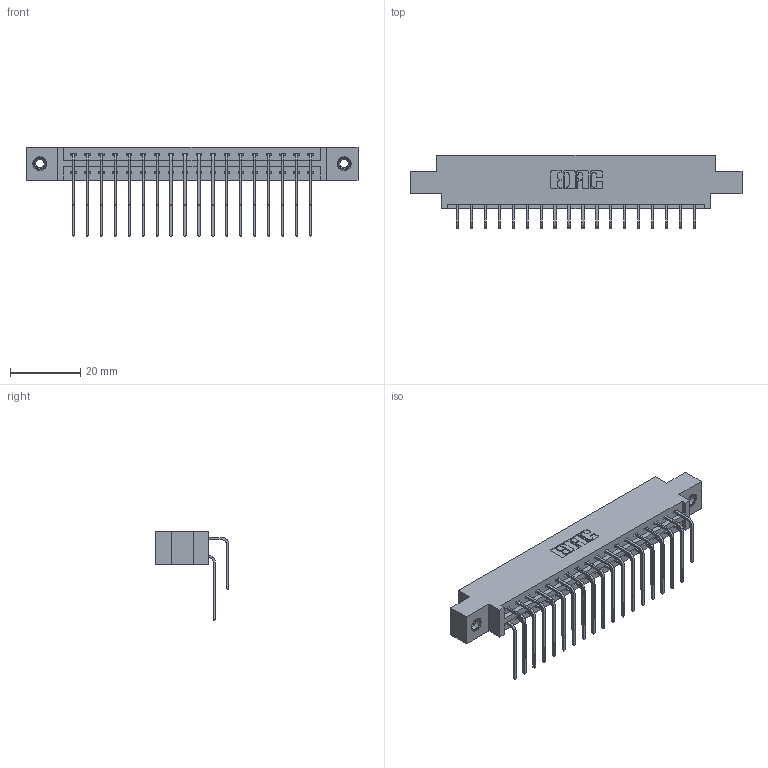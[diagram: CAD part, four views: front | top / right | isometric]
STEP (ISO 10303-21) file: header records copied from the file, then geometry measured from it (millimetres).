
FILE_DESCRIPTION (( 'STEP AP203' ), '1' );
FILE_NAME ('337-036-559-807.STEP', '2018-08-08T00:28:37', ( '' ), ( '' ), 'SwSTEP 2.0', 'SolidWorks 2016', '' );
FILE_SCHEMA (( 'CONFIG_CONTROL_DESIGN' ));
Length unit declared in the file: inch
Products named in the file (5): 337 Part_0.170 Offset - 0.156 Dia-TI; 345-292-001_558 559 Tail - 1; 345-292-001_559 Tail - 2; 345-250-001_345-250-005-103; 337-036-559-807
Assembly tree (39 placements, depth 2):
  337-036-559-807
    337 Part_0.170 Offset - 0.156 Dia-TI
    345-292-001_558 559 Tail - 1  x18
    345-292-001_559 Tail - 2  x18
    345-250-001_345-250-005-103  x2
Bounding box: 94.34 x 20.9 x 25.53 mm (x, y, z)
Volume: 9699 mm3; surface area: 11918.2 mm2
Topology: 39 solids, 39 shells, 2194 faces, 6471 edges, 4258 vertices
Faces by surface type: plane 1546, cylinder 632, cone 12, torus 4
Entity records: 20162 total; most frequent: CARTESIAN_POINT 3444, ORIENTED_EDGE 3322, DIRECTION 2987, EDGE_CURVE 1661, LINE 1473, VECTOR 1473, VERTEX_POINT 1100, AXIS2_PLACEMENT_3D 757
